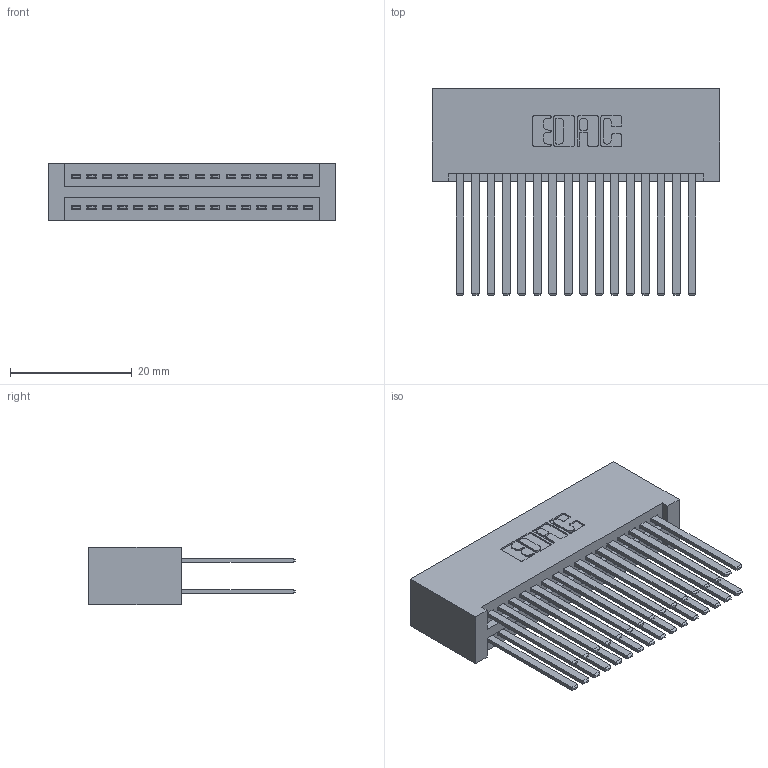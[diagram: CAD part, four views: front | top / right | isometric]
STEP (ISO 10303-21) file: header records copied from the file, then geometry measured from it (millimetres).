
FILE_DESCRIPTION (( 'STEP AP203' ), '1' );
FILE_NAME ('345-032-544-201.STEP', '2018-08-24T07:48:29', ( '' ), ( '' ), 'SwSTEP 2.0', 'SolidWorks 2016', '' );
FILE_SCHEMA (( 'CONFIG_CONTROL_DESIGN' ));
Length unit declared in the file: inch
Products named in the file (3): 345 Part_No Mounting Lugs; 345-292-001_345-293-144; 345-032-544-201
Assembly tree (33 placements, depth 2):
  345-032-544-201
    345 Part_No Mounting Lugs
    345-292-001_345-293-144  x32
Bounding box: 47.24 x 33.96 x 9.4 mm (x, y, z)
Volume: 5412.5 mm3; surface area: 9115 mm2
Topology: 33 solids, 33 shells, 1526 faces, 4509 edges, 2962 vertices
Faces by surface type: plane 1004, cylinder 522
Entity records: 15593 total; most frequent: CARTESIAN_POINT 2636, ORIENTED_EDGE 2570, DIRECTION 2349, EDGE_CURVE 1285, VECTOR 1101, LINE 1101, VERTEX_POINT 854, AXIS2_PLACEMENT_3D 624
